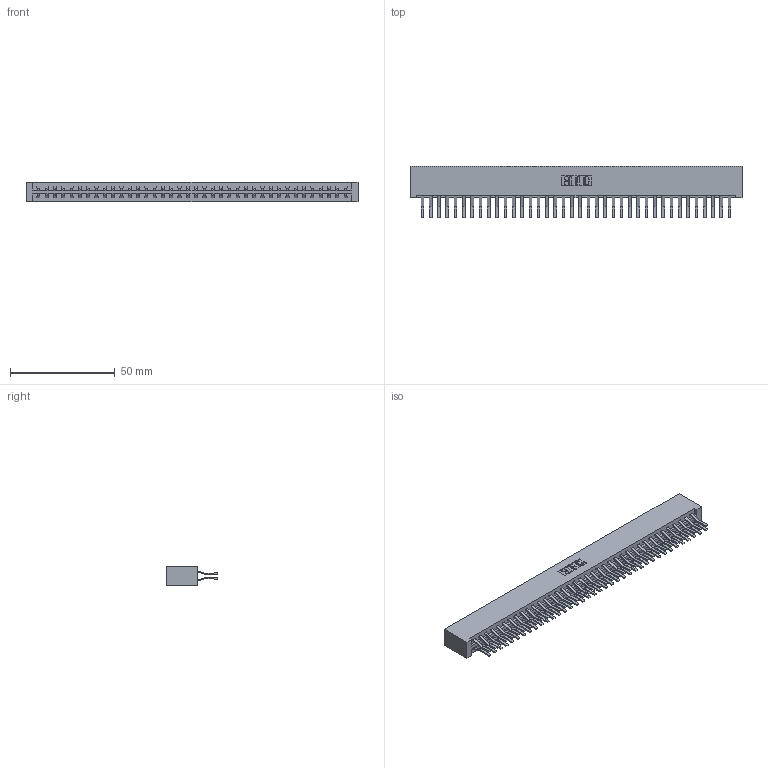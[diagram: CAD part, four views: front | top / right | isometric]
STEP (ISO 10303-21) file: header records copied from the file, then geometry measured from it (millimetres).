
FILE_DESCRIPTION (( 'STEP AP203' ), '1' );
FILE_NAME ('337-076-560-201.STEP', '2018-08-12T15:03:08', ( '' ), ( '' ), 'SwSTEP 2.0', 'SolidWorks 2016', '' );
FILE_SCHEMA (( 'CONFIG_CONTROL_DESIGN' ));
Length unit declared in the file: inch
Products named in the file (3): 337 Part_No Mounting Lugs; 345-292-001_560 Tail; 337-076-560-201
Assembly tree (77 placements, depth 2):
  337-076-560-201
    337 Part_No Mounting Lugs
    345-292-001_560 Tail  x76
Bounding box: 158.45 x 24.78 x 9.4 mm (x, y, z)
Volume: 17903.9 mm3; surface area: 21699.4 mm2
Topology: 77 solids, 77 shells, 4362 faces, 12979 edges, 8550 vertices
Faces by surface type: plane 2954, cylinder 1408
Entity records: 29791 total; most frequent: CARTESIAN_POINT 5022, ORIENTED_EDGE 4958, DIRECTION 4275, EDGE_CURVE 2479, VECTOR 2355, LINE 2355, VERTEX_POINT 1650, AXIS2_PLACEMENT_3D 960
